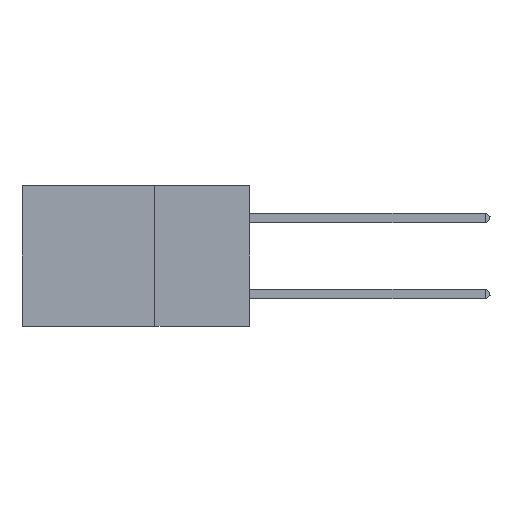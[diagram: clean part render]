
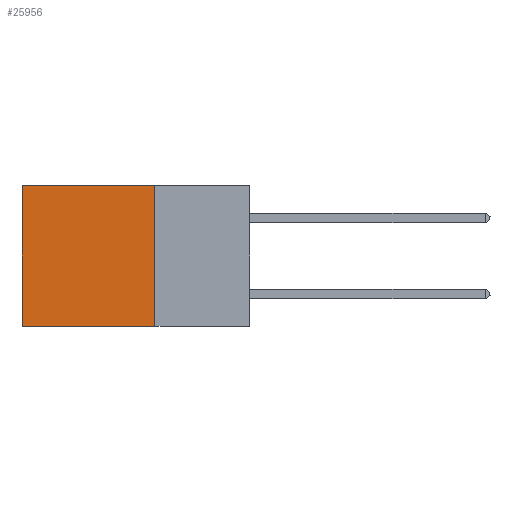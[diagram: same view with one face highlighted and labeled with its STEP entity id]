
A CAD part, left-side view. The second image highlights one B-rep face of the part: STEP entity #25956.
In plain terms, the highlighted planar face has unit normal (-1, 0, 0).
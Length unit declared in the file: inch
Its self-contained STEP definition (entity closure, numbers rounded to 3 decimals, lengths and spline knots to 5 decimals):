
#3 = CARTESIAN_POINT ( 'NONE',  ( 0.2875, 0.6, 0. ) ) ;
#134 = LINE ( 'NONE', #9771, #15762 ) ;
#158 = CARTESIAN_POINT ( 'NONE',  ( 0.2875, 0.25, 0. ) ) ;
#1827 = LINE ( 'NONE', #3, #18089 ) ;
#2285 = AXIS2_PLACEMENT_3D ( 'NONE', #22373, #16301, #4144 ) ;
#3297 = EDGE_CURVE ( 'NONE', #12207, #20888, #8133, .T. ) ;
#3538 = ORIENTED_EDGE ( 'NONE', *, *, #4337, .F. ) ;
#3721 = CARTESIAN_POINT ( 'NONE',  ( 0.2875, 0.6, 0. ) ) ;
#4144 = DIRECTION ( 'NONE',  ( 0., 0., -1. ) ) ;
#4337 = EDGE_CURVE ( 'NONE', #10704, #12207, #134, .T. ) ;
#6860 = VECTOR ( 'NONE', #8860, 39.37008 ) ;
#8133 = LINE ( 'NONE', #18998, #6860 ) ;
#8151 = DIRECTION ( 'NONE',  ( 0., 0., -1. ) ) ;
#8860 = DIRECTION ( 'NONE',  ( 0., 1., 0. ) ) ;
#9296 = FACE_OUTER_BOUND ( 'NONE', #11662, .T. ) ;
#9771 = CARTESIAN_POINT ( 'NONE',  ( 0.2875, 0.25, 0. ) ) ;
#10149 = DIRECTION ( 'NONE',  ( 0., 1., 0. ) ) ;
#10704 = VERTEX_POINT ( 'NONE', #158 ) ;
#11064 = ORIENTED_EDGE ( 'NONE', *, *, #20896, .T. ) ;
#11185 = VERTEX_POINT ( 'NONE', #3721 ) ;
#11662 = EDGE_LOOP ( 'NONE', ( #11064, #15130, #3538, #25400 ) ) ;
#12207 = VERTEX_POINT ( 'NONE', #15156 ) ;
#12471 = VECTOR ( 'NONE', #10149, 39.37008 ) ;
#13856 = DIRECTION ( 'NONE',  ( 0., 0., -1. ) ) ;
#15130 = ORIENTED_EDGE ( 'NONE', *, *, #3297, .F. ) ;
#15140 = EDGE_CURVE ( 'NONE', #10704, #11185, #22034, .T. ) ;
#15156 = CARTESIAN_POINT ( 'NONE',  ( 0.2875, 0.25, -0.37 ) ) ;
#15762 = VECTOR ( 'NONE', #13856, 39.37008 ) ;
#16301 = DIRECTION ( 'NONE',  ( 1., 0., 0. ) ) ;
#18089 = VECTOR ( 'NONE', #8151, 39.37008 ) ;
#18998 = CARTESIAN_POINT ( 'NONE',  ( 0.2875, 0.25, -0.37 ) ) ;
#20888 = VERTEX_POINT ( 'NONE', #22374 ) ;
#20896 = EDGE_CURVE ( 'NONE', #11185, #20888, #1827, .T. ) ;
#22034 = LINE ( 'NONE', #24393, #12471 ) ;
#22373 = CARTESIAN_POINT ( 'NONE',  ( 0.2875, 0.25, 0. ) ) ;
#22374 = CARTESIAN_POINT ( 'NONE',  ( 0.2875, 0.6, -0.37 ) ) ;
#24393 = CARTESIAN_POINT ( 'NONE',  ( 0.2875, 0.25, 0. ) ) ;
#25400 = ORIENTED_EDGE ( 'NONE', *, *, #15140, .T. ) ;
#25956 = ADVANCED_FACE ( 'NONE', ( #9296 ), #26382, .F. ) ;
#26382 = PLANE ( 'NONE',  #2285 ) ;
